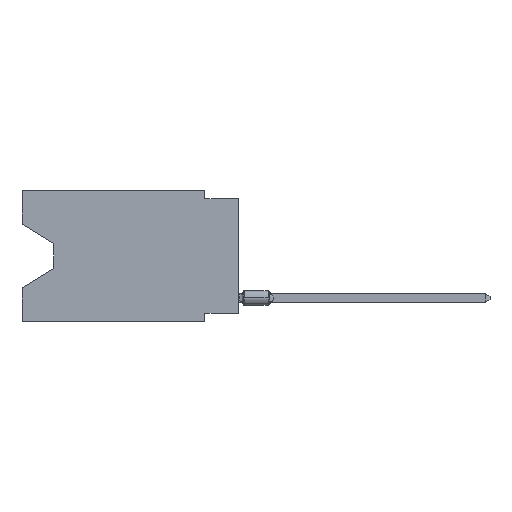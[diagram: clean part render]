
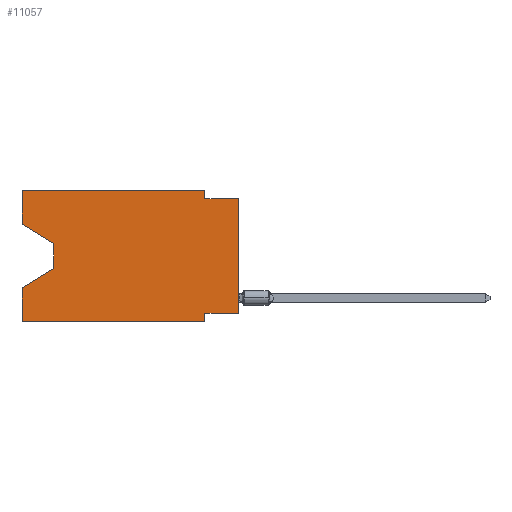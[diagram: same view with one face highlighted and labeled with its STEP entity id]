
A CAD part, left-side view. The second image highlights one B-rep face of the part: STEP entity #11057.
In plain terms, the highlighted planar face has unit normal (-1, 0, 0).
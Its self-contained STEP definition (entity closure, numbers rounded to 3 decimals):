
#31 = DIRECTION ( 'NONE',  ( 0., -0.855, -0.519 ) ) ;
#562 = EDGE_CURVE ( 'NONE', #2384, #21028, #22127, .T. ) ;
#1142 = EDGE_CURVE ( 'NONE', #2822, #25148, #8156, .T. ) ;
#1320 = CARTESIAN_POINT ( 'NONE',  ( 0., 2.54, -9.906 ) ) ;
#2222 = VERTEX_POINT ( 'NONE', #8916 ) ;
#2384 = VERTEX_POINT ( 'NONE', #26199 ) ;
#2787 = EDGE_CURVE ( 'NONE', #24620, #13777, #17594, .T. ) ;
#2822 = VERTEX_POINT ( 'NONE', #5743 ) ;
#2824 = PLANE ( 'NONE',  #6325 ) ;
#3091 = EDGE_CURVE ( 'NONE', #26858, #10355, #17049, .T. ) ;
#3695 = ORIENTED_EDGE ( 'NONE', *, *, #20540, .F. ) ;
#4322 = CARTESIAN_POINT ( 'NONE',  ( 0., 16.383, -2.546 ) ) ;
#4329 = DIRECTION ( 'NONE',  ( 0., 0., -1. ) ) ;
#4712 = VECTOR ( 'NONE', #4329, 1000. ) ;
#4941 = VERTEX_POINT ( 'NONE', #7732 ) ;
#5089 = VECTOR ( 'NONE', #31, 1000. ) ;
#5400 = DIRECTION ( 'NONE',  ( 0., 1., 0. ) ) ;
#5462 = LINE ( 'NONE', #27827, #10116 ) ;
#5609 = DIRECTION ( 'NONE',  ( 0., 0., -1. ) ) ;
#5743 = CARTESIAN_POINT ( 'NONE',  ( 0., 16.383, -9.906 ) ) ;
#5770 = CARTESIAN_POINT ( 'NONE',  ( 0., 0., 0. ) ) ;
#6027 = DIRECTION ( 'NONE',  ( 0., 0., -1. ) ) ;
#6325 = AXIS2_PLACEMENT_3D ( 'NONE', #28132, #25910, #9623 ) ;
#7607 = ORIENTED_EDGE ( 'NONE', *, *, #18939, .F. ) ;
#7656 = CARTESIAN_POINT ( 'NONE',  ( 0., 16.383, 0. ) ) ;
#7688 = CARTESIAN_POINT ( 'NONE',  ( 0., 16.383, 0. ) ) ;
#7732 = CARTESIAN_POINT ( 'NONE',  ( 0., 2.54, 0. ) ) ;
#8156 = LINE ( 'NONE', #10528, #9201 ) ;
#8808 = DIRECTION ( 'NONE',  ( 0., -1., 0. ) ) ;
#8916 = CARTESIAN_POINT ( 'NONE',  ( 0., 13.97, -5.893 ) ) ;
#8972 = VERTEX_POINT ( 'NONE', #23752 ) ;
#9182 = VECTOR ( 'NONE', #19918, 1000. ) ;
#9201 = VECTOR ( 'NONE', #14847, 1000. ) ;
#9247 = VECTOR ( 'NONE', #5400, 1000. ) ;
#9253 = CARTESIAN_POINT ( 'NONE',  ( 0., 16.383, -7.36 ) ) ;
#9623 = DIRECTION ( 'NONE',  ( 0., 0., -1. ) ) ;
#9858 = CARTESIAN_POINT ( 'NONE',  ( 0., 0., -9.271 ) ) ;
#10116 = VECTOR ( 'NONE', #5609, 1000. ) ;
#10355 = VERTEX_POINT ( 'NONE', #20248 ) ;
#10493 = VECTOR ( 'NONE', #21625, 1000. ) ;
#10528 = CARTESIAN_POINT ( 'NONE',  ( 0., 16.383, 0. ) ) ;
#10820 = VECTOR ( 'NONE', #21652, 1000. ) ;
#11057 = ADVANCED_FACE ( 'NONE', ( #23086 ), #2824, .F. ) ;
#11430 = VECTOR ( 'NONE', #6027, 1000. ) ;
#12297 = LINE ( 'NONE', #7688, #23184 ) ;
#12395 = CARTESIAN_POINT ( 'NONE',  ( 0., 13.97, -5.893 ) ) ;
#12904 = LINE ( 'NONE', #22085, #10820 ) ;
#13360 = EDGE_CURVE ( 'NONE', #15341, #2222, #5462, .T. ) ;
#13777 = VERTEX_POINT ( 'NONE', #28927 ) ;
#14811 = DIRECTION ( 'NONE',  ( 0., -1., 0. ) ) ;
#14847 = DIRECTION ( 'NONE',  ( 0., 0., 1. ) ) ;
#14998 = ORIENTED_EDGE ( 'NONE', *, *, #3091, .T. ) ;
#15246 = ORIENTED_EDGE ( 'NONE', *, *, #18755, .F. ) ;
#15341 = VERTEX_POINT ( 'NONE', #18809 ) ;
#15583 = LINE ( 'NONE', #4322, #5089 ) ;
#15919 = ORIENTED_EDGE ( 'NONE', *, *, #26293, .F. ) ;
#15942 = EDGE_CURVE ( 'NONE', #2822, #13777, #27015, .T. ) ;
#16525 = LINE ( 'NONE', #9858, #9247 ) ;
#16783 = VECTOR ( 'NONE', #21413, 1000. ) ;
#16900 = ORIENTED_EDGE ( 'NONE', *, *, #13360, .T. ) ;
#17049 = LINE ( 'NONE', #5770, #10493 ) ;
#17594 = LINE ( 'NONE', #1320, #11430 ) ;
#18116 = ORIENTED_EDGE ( 'NONE', *, *, #20355, .T. ) ;
#18554 = ORIENTED_EDGE ( 'NONE', *, *, #27521, .T. ) ;
#18755 = EDGE_CURVE ( 'NONE', #8972, #10355, #12904, .T. ) ;
#18809 = CARTESIAN_POINT ( 'NONE',  ( 0., 13.97, -4.013 ) ) ;
#18939 = EDGE_CURVE ( 'NONE', #4941, #8972, #22367, .T. ) ;
#19491 = LINE ( 'NONE', #12395, #16783 ) ;
#19918 = DIRECTION ( 'NONE',  ( 0., 0., 1. ) ) ;
#20176 = CARTESIAN_POINT ( 'NONE',  ( 0., 2.54, 0. ) ) ;
#20248 = CARTESIAN_POINT ( 'NONE',  ( 0., 0., -0.635 ) ) ;
#20355 = EDGE_CURVE ( 'NONE', #2384, #15341, #15583, .T. ) ;
#20470 = CARTESIAN_POINT ( 'NONE',  ( 0., 0., -9.271 ) ) ;
#20540 = EDGE_CURVE ( 'NONE', #21028, #4941, #12297, .T. ) ;
#20623 = VECTOR ( 'NONE', #8808, 1000. ) ;
#21028 = VERTEX_POINT ( 'NONE', #7656 ) ;
#21413 = DIRECTION ( 'NONE',  ( 0., 0.855, -0.519 ) ) ;
#21625 = DIRECTION ( 'NONE',  ( 0., 0., 1. ) ) ;
#21652 = DIRECTION ( 'NONE',  ( 0., -1., 0. ) ) ;
#22085 = CARTESIAN_POINT ( 'NONE',  ( 0., 0., -0.635 ) ) ;
#22127 = LINE ( 'NONE', #28484, #9182 ) ;
#22367 = LINE ( 'NONE', #20176, #4712 ) ;
#23086 = FACE_OUTER_BOUND ( 'NONE', #23376, .T. ) ;
#23184 = VECTOR ( 'NONE', #14811, 1000. ) ;
#23376 = EDGE_LOOP ( 'NONE', ( #18116, #16900, #18554, #26097, #24013, #23878, #15919, #14998, #15246, #7607, #3695, #23529 ) ) ;
#23529 = ORIENTED_EDGE ( 'NONE', *, *, #562, .F. ) ;
#23752 = CARTESIAN_POINT ( 'NONE',  ( 0., 2.54, -0.635 ) ) ;
#23878 = ORIENTED_EDGE ( 'NONE', *, *, #2787, .F. ) ;
#24013 = ORIENTED_EDGE ( 'NONE', *, *, #15942, .T. ) ;
#24620 = VERTEX_POINT ( 'NONE', #24834 ) ;
#24834 = CARTESIAN_POINT ( 'NONE',  ( 0., 2.54, -9.271 ) ) ;
#25148 = VERTEX_POINT ( 'NONE', #9253 ) ;
#25910 = DIRECTION ( 'NONE',  ( 1., 0., 0. ) ) ;
#26097 = ORIENTED_EDGE ( 'NONE', *, *, #1142, .F. ) ;
#26199 = CARTESIAN_POINT ( 'NONE',  ( 0., 16.383, -2.546 ) ) ;
#26293 = EDGE_CURVE ( 'NONE', #26858, #24620, #16525, .T. ) ;
#26858 = VERTEX_POINT ( 'NONE', #20470 ) ;
#27015 = LINE ( 'NONE', #29077, #20623 ) ;
#27521 = EDGE_CURVE ( 'NONE', #2222, #25148, #19491, .T. ) ;
#27827 = CARTESIAN_POINT ( 'NONE',  ( 0., 13.97, -4.013 ) ) ;
#28132 = CARTESIAN_POINT ( 'NONE',  ( 0., 16.383, 0. ) ) ;
#28484 = CARTESIAN_POINT ( 'NONE',  ( 0., 16.383, 0. ) ) ;
#28927 = CARTESIAN_POINT ( 'NONE',  ( 0., 2.54, -9.906 ) ) ;
#29077 = CARTESIAN_POINT ( 'NONE',  ( 0., 16.383, -9.906 ) ) ;
